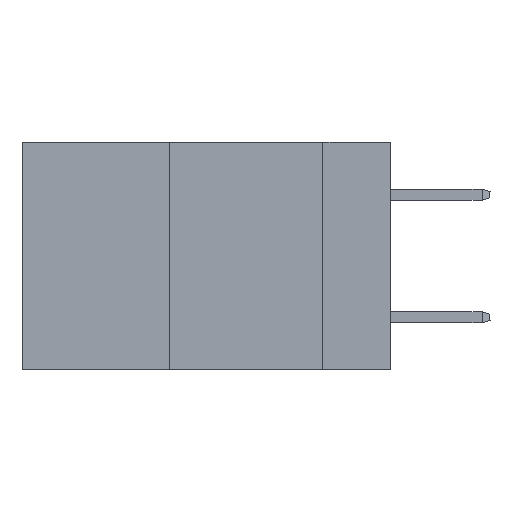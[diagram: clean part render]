
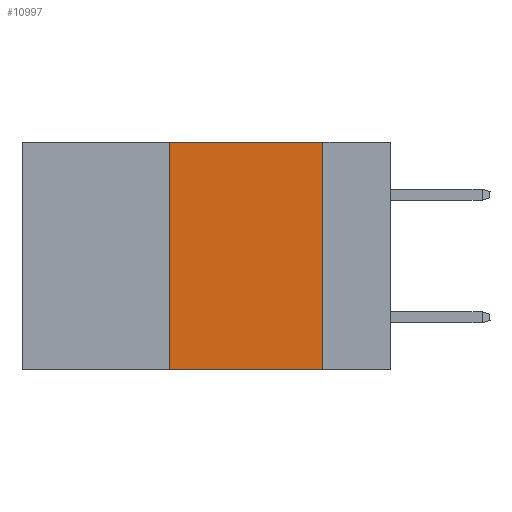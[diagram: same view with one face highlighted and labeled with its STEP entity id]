
A CAD part, left-side view. The second image highlights one B-rep face of the part: STEP entity #10997.
In plain terms, the highlighted planar face has unit normal (-1, 0, 0).
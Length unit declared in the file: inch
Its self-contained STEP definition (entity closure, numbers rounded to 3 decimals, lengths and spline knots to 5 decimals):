
#776 = ORIENTED_EDGE ( 'NONE', *, *, #1260, .T. ) ;
#1164 = CARTESIAN_POINT ( 'NONE',  ( 0., 0.11, -0.37 ) ) ;
#1260 = EDGE_CURVE ( 'NONE', #3474, #9068, #3196, .T. ) ;
#1297 = LINE ( 'NONE', #12568, #1840 ) ;
#1471 = VECTOR ( 'NONE', #20953, 39.37008 ) ;
#1755 = EDGE_CURVE ( 'NONE', #6716, #9068, #1297, .T. ) ;
#1759 = DIRECTION ( 'NONE',  ( 0., -1., 0. ) ) ;
#1840 = VECTOR ( 'NONE', #8365, 39.37008 ) ;
#3196 = LINE ( 'NONE', #5638, #16008 ) ;
#3474 = VERTEX_POINT ( 'NONE', #5273 ) ;
#4708 = EDGE_LOOP ( 'NONE', ( #7414, #11860, #7430, #776 ) ) ;
#5273 = CARTESIAN_POINT ( 'NONE',  ( 0., 0.36, -0.37 ) ) ;
#5638 = CARTESIAN_POINT ( 'NONE',  ( 0., 0.6, -0.37 ) ) ;
#5863 = VECTOR ( 'NONE', #1759, 39.37008 ) ;
#6698 = CARTESIAN_POINT ( 'NONE',  ( 0., 0.6, 0. ) ) ;
#6716 = VERTEX_POINT ( 'NONE', #19361 ) ;
#7414 = ORIENTED_EDGE ( 'NONE', *, *, #1755, .F. ) ;
#7430 = ORIENTED_EDGE ( 'NONE', *, *, #11372, .F. ) ;
#7452 = DIRECTION ( 'NONE',  ( 0., -1., 0. ) ) ;
#8365 = DIRECTION ( 'NONE',  ( 0., 0., -1. ) ) ;
#9068 = VERTEX_POINT ( 'NONE', #1164 ) ;
#10448 = LINE ( 'NONE', #6698, #5863 ) ;
#10632 = CARTESIAN_POINT ( 'NONE',  ( 0., 0.6, 0. ) ) ;
#10997 = ADVANCED_FACE ( 'NONE', ( #20747 ), #12552, .F. ) ;
#11063 = CARTESIAN_POINT ( 'NONE',  ( 0., 0.36, 0. ) ) ;
#11372 = EDGE_CURVE ( 'NONE', #3474, #15524, #16145, .T. ) ;
#11860 = ORIENTED_EDGE ( 'NONE', *, *, #17245, .F. ) ;
#12552 = PLANE ( 'NONE',  #16671 ) ;
#12568 = CARTESIAN_POINT ( 'NONE',  ( 0., 0.11, 0. ) ) ;
#14136 = DIRECTION ( 'NONE',  ( 0., 0., -1. ) ) ;
#14205 = DIRECTION ( 'NONE',  ( 1., 0., 0. ) ) ;
#15524 = VERTEX_POINT ( 'NONE', #11063 ) ;
#16008 = VECTOR ( 'NONE', #7452, 39.37008 ) ;
#16145 = LINE ( 'NONE', #19239, #1471 ) ;
#16671 = AXIS2_PLACEMENT_3D ( 'NONE', #10632, #14205, #14136 ) ;
#17245 = EDGE_CURVE ( 'NONE', #15524, #6716, #10448, .T. ) ;
#19239 = CARTESIAN_POINT ( 'NONE',  ( 0., 0.36, 0. ) ) ;
#19361 = CARTESIAN_POINT ( 'NONE',  ( 0., 0.11, 0. ) ) ;
#20747 = FACE_OUTER_BOUND ( 'NONE', #4708, .T. ) ;
#20953 = DIRECTION ( 'NONE',  ( 0., 0., 1. ) ) ;
